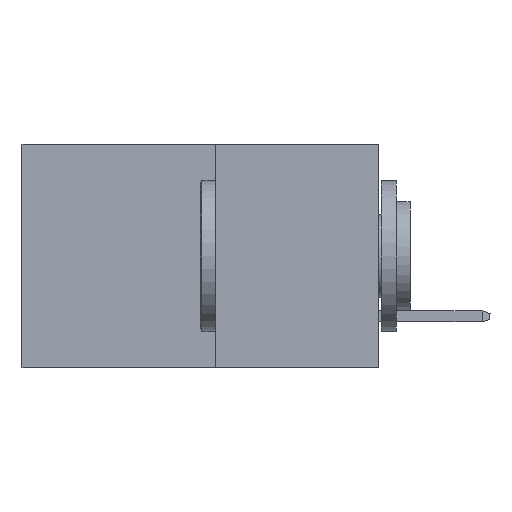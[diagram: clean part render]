
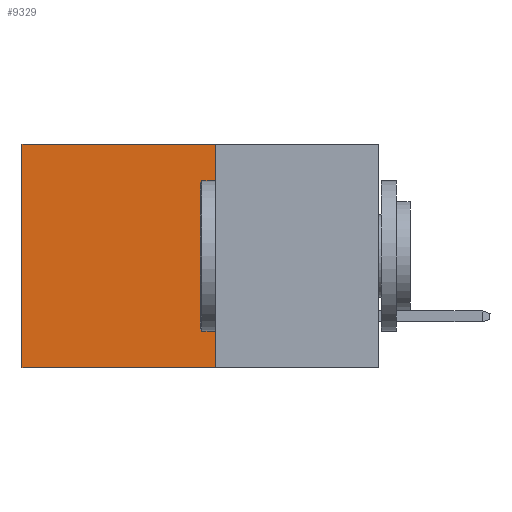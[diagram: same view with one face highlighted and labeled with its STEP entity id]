
A CAD part, left-side view. The second image highlights one B-rep face of the part: STEP entity #9329.
In plain terms, the highlighted planar face has unit normal (-1, 0, 0).
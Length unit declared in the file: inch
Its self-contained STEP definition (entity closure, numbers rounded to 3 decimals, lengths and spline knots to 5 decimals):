
#1277 = FACE_OUTER_BOUND ( 'NONE', #5194, .T. ) ;
#1873 = CARTESIAN_POINT ( 'NONE',  ( 0.277, 0.27, -0.37 ) ) ;
#2671 = CARTESIAN_POINT ( 'NONE',  ( 0.277, 0.27, -0.37 ) ) ;
#2734 = CARTESIAN_POINT ( 'NONE',  ( 0.277, 0.27, 0. ) ) ;
#3101 = CARTESIAN_POINT ( 'NONE',  ( 0.277, 0.59, -0.37 ) ) ;
#3157 = DIRECTION ( 'NONE',  ( 0., 0., -1. ) ) ;
#3923 = EDGE_CURVE ( 'NONE', #8409, #8582, #9242, .T. ) ;
#4163 = ORIENTED_EDGE ( 'NONE', *, *, #4590, .T. ) ;
#4182 = ORIENTED_EDGE ( 'NONE', *, *, #3923, .F. ) ;
#4196 = ORIENTED_EDGE ( 'NONE', *, *, #8322, .F. ) ;
#4218 = ORIENTED_EDGE ( 'NONE', *, *, #7007, .T. ) ;
#4384 = VECTOR ( 'NONE', #6518, 39.37008 ) ;
#4413 = PLANE ( 'NONE',  #4433 ) ;
#4433 = AXIS2_PLACEMENT_3D ( 'NONE', #10351, #5308, #11162 ) ;
#4590 = EDGE_CURVE ( 'NONE', #8787, #8582, #5253, .T. ) ;
#4714 = VECTOR ( 'NONE', #3157, 39.37008 ) ;
#4803 = CARTESIAN_POINT ( 'NONE',  ( 0.277, 0.27, 0. ) ) ;
#5194 = EDGE_LOOP ( 'NONE', ( #4163, #4182, #4196, #4218 ) ) ;
#5253 = LINE ( 'NONE', #3101, #4714 ) ;
#5308 = DIRECTION ( 'NONE',  ( 1., 0., 0. ) ) ;
#6518 = DIRECTION ( 'NONE',  ( 0., 1., 0. ) ) ;
#7007 = EDGE_CURVE ( 'NONE', #7511, #8787, #11114, .T. ) ;
#7143 = LINE ( 'NONE', #2671, #9387 ) ;
#7281 = VECTOR ( 'NONE', #8537, 39.37008 ) ;
#7511 = VERTEX_POINT ( 'NONE', #2734 ) ;
#7954 = DIRECTION ( 'NONE',  ( 0., 0., -1. ) ) ;
#8246 = CARTESIAN_POINT ( 'NONE',  ( 0.277, 0.59, -0.37 ) ) ;
#8322 = EDGE_CURVE ( 'NONE', #7511, #8409, #7143, .T. ) ;
#8409 = VERTEX_POINT ( 'NONE', #1873 ) ;
#8537 = DIRECTION ( 'NONE',  ( 0., 1., 0. ) ) ;
#8545 = CARTESIAN_POINT ( 'NONE',  ( 0.277, 0.27, -0.37 ) ) ;
#8582 = VERTEX_POINT ( 'NONE', #8246 ) ;
#8787 = VERTEX_POINT ( 'NONE', #9683 ) ;
#9242 = LINE ( 'NONE', #8545, #7281 ) ;
#9329 = ADVANCED_FACE ( 'NONE', ( #1277 ), #4413, .F. ) ;
#9387 = VECTOR ( 'NONE', #7954, 39.37008 ) ;
#9683 = CARTESIAN_POINT ( 'NONE',  ( 0.277, 0.59, 0. ) ) ;
#10351 = CARTESIAN_POINT ( 'NONE',  ( 0.277, 0.27, -0.37 ) ) ;
#11114 = LINE ( 'NONE', #4803, #4384 ) ;
#11162 = DIRECTION ( 'NONE',  ( 0., 0., -1. ) ) ;
